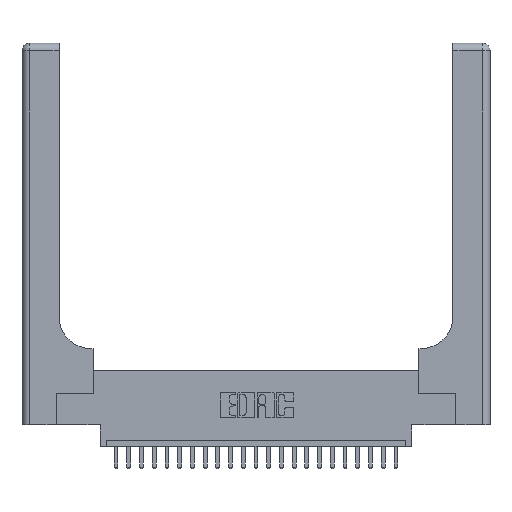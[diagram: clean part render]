
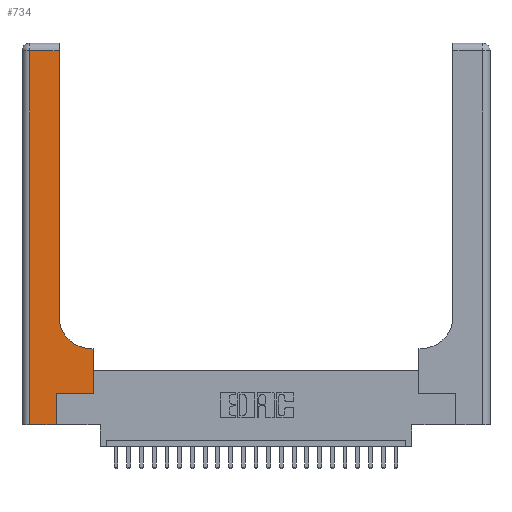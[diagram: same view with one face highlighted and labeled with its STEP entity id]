
A CAD part, top view. The second image highlights one B-rep face of the part: STEP entity #734.
In plain terms, the highlighted planar face has unit normal (0, 0, 1).
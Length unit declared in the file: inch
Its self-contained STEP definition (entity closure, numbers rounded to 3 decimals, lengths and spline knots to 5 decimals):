
#443 = ORIENTED_EDGE ( 'NONE', *, *, #13530, .T. ) ;
#529 = VECTOR ( 'NONE', #8197, 39.37008 ) ;
#697 = ORIENTED_EDGE ( 'NONE', *, *, #7268, .T. ) ;
#734 = ADVANCED_FACE ( 'NONE', ( #11879 ), #20268, .F. ) ;
#1260 = VERTEX_POINT ( 'NONE', #9228 ) ;
#1275 = DIRECTION ( 'NONE',  ( -1., 0., 0. ) ) ;
#1363 = ORIENTED_EDGE ( 'NONE', *, *, #17161, .T. ) ;
#1904 = EDGE_CURVE ( 'NONE', #24239, #1260, #17369, .T. ) ;
#2392 = CARTESIAN_POINT ( 'NONE',  ( 0.5415, 0.6, 0.37 ) ) ;
#2810 = CARTESIAN_POINT ( 'NONE',  ( 0.06, 3., 0.37 ) ) ;
#2931 = LINE ( 'NONE', #3161, #11792 ) ;
#3161 = CARTESIAN_POINT ( 'NONE',  ( 0., 0., 0.37 ) ) ;
#3208 = CARTESIAN_POINT ( 'NONE',  ( 0.5585, 0.6, 0.37 ) ) ;
#3316 = DIRECTION ( 'NONE',  ( 0., 0., -1. ) ) ;
#3609 = VECTOR ( 'NONE', #6597, 39.37008 ) ;
#4708 = ORIENTED_EDGE ( 'NONE', *, *, #6054, .T. ) ;
#4972 = ORIENTED_EDGE ( 'NONE', *, *, #24014, .T. ) ;
#5376 = CARTESIAN_POINT ( 'NONE',  ( 0.269, 0., 0.37 ) ) ;
#5452 = LINE ( 'NONE', #2810, #3609 ) ;
#5463 = CARTESIAN_POINT ( 'NONE',  ( 0.5585, 0.25, 0.37 ) ) ;
#6054 = EDGE_CURVE ( 'NONE', #8722, #24239, #10647, .T. ) ;
#6098 = LINE ( 'NONE', #8687, #15873 ) ;
#6276 = VECTOR ( 'NONE', #16962, 39.37008 ) ;
#6362 = VERTEX_POINT ( 'NONE', #12364 ) ;
#6374 = DIRECTION ( 'NONE',  ( 0., 0., -1. ) ) ;
#6597 = DIRECTION ( 'NONE',  ( 0., -1., 0. ) ) ;
#6871 = CARTESIAN_POINT ( 'NONE',  ( 0.269, 0., 0.37 ) ) ;
#6943 = CARTESIAN_POINT ( 'NONE',  ( 0.269, 0.25, 0.37 ) ) ;
#6971 = EDGE_CURVE ( 'NONE', #22836, #15444, #21625, .T. ) ;
#7268 = EDGE_CURVE ( 'NONE', #15444, #16836, #19467, .T. ) ;
#7806 = ORIENTED_EDGE ( 'NONE', *, *, #6971, .T. ) ;
#8197 = DIRECTION ( 'NONE',  ( -1., 0., 0. ) ) ;
#8687 = CARTESIAN_POINT ( 'NONE',  ( 0., 2.94, 0.37 ) ) ;
#8722 = VERTEX_POINT ( 'NONE', #3208 ) ;
#8725 = DIRECTION ( 'NONE',  ( 1., 0., 0. ) ) ;
#9228 = CARTESIAN_POINT ( 'NONE',  ( 0.2915, 0.85, 0.37 ) ) ;
#9913 = VERTEX_POINT ( 'NONE', #21121 ) ;
#10647 = LINE ( 'NONE', #19911, #529 ) ;
#10932 = CARTESIAN_POINT ( 'NONE',  ( 0., 3., 0.37 ) ) ;
#11119 = CARTESIAN_POINT ( 'NONE',  ( 0.2915, 3., 0.37 ) ) ;
#11792 = VECTOR ( 'NONE', #20704, 39.37008 ) ;
#11879 = FACE_OUTER_BOUND ( 'NONE', #21944, .T. ) ;
#11937 = ORIENTED_EDGE ( 'NONE', *, *, #1904, .T. ) ;
#12273 = DIRECTION ( 'NONE',  ( 0., 1., 0. ) ) ;
#12331 = CARTESIAN_POINT ( 'NONE',  ( 0.5415, 0.85, 0.37 ) ) ;
#12364 = CARTESIAN_POINT ( 'NONE',  ( 0.06, 0., 0.37 ) ) ;
#13530 = EDGE_CURVE ( 'NONE', #9913, #6362, #5452, .T. ) ;
#13837 = VECTOR ( 'NONE', #12273, 39.37008 ) ;
#15166 = LINE ( 'NONE', #11119, #6276 ) ;
#15444 = VERTEX_POINT ( 'NONE', #22569 ) ;
#15873 = VECTOR ( 'NONE', #22297, 39.37008 ) ;
#16594 = ORIENTED_EDGE ( 'NONE', *, *, #21453, .T. ) ;
#16836 = VERTEX_POINT ( 'NONE', #5463 ) ;
#16962 = DIRECTION ( 'NONE',  ( 0., 1., 0. ) ) ;
#17161 = EDGE_CURVE ( 'NONE', #16836, #8722, #17829, .T. ) ;
#17369 = CIRCLE ( 'NONE', #18002, 0.25 ) ;
#17829 = LINE ( 'NONE', #20081, #13837 ) ;
#18002 = AXIS2_PLACEMENT_3D ( 'NONE', #12331, #6374, #22186 ) ;
#19467 = LINE ( 'NONE', #6943, #22539 ) ;
#19479 = CARTESIAN_POINT ( 'NONE',  ( 0.2915, 2.94, 0.37 ) ) ;
#19911 = CARTESIAN_POINT ( 'NONE',  ( 0.2915, 0.6, 0.37 ) ) ;
#20023 = EDGE_CURVE ( 'NONE', #22973, #9913, #6098, .T. ) ;
#20081 = CARTESIAN_POINT ( 'NONE',  ( 0.5585, 0.25, 0.37 ) ) ;
#20268 = PLANE ( 'NONE',  #24662 ) ;
#20704 = DIRECTION ( 'NONE',  ( 1., 0., 0. ) ) ;
#21121 = CARTESIAN_POINT ( 'NONE',  ( 0.06, 2.94, 0.37 ) ) ;
#21177 = ORIENTED_EDGE ( 'NONE', *, *, #20023, .T. ) ;
#21453 = EDGE_CURVE ( 'NONE', #6362, #22836, #2931, .T. ) ;
#21625 = LINE ( 'NONE', #6871, #23461 ) ;
#21944 = EDGE_LOOP ( 'NONE', ( #4972, #21177, #443, #16594, #7806, #697, #1363, #4708, #11937 ) ) ;
#22186 = DIRECTION ( 'NONE',  ( 1., 0., 0. ) ) ;
#22297 = DIRECTION ( 'NONE',  ( -1., 0., 0. ) ) ;
#22539 = VECTOR ( 'NONE', #8725, 39.37008 ) ;
#22569 = CARTESIAN_POINT ( 'NONE',  ( 0.269, 0.25, 0.37 ) ) ;
#22679 = DIRECTION ( 'NONE',  ( 0., 1., 0. ) ) ;
#22836 = VERTEX_POINT ( 'NONE', #5376 ) ;
#22973 = VERTEX_POINT ( 'NONE', #19479 ) ;
#23461 = VECTOR ( 'NONE', #22679, 39.37008 ) ;
#24014 = EDGE_CURVE ( 'NONE', #1260, #22973, #15166, .T. ) ;
#24239 = VERTEX_POINT ( 'NONE', #2392 ) ;
#24662 = AXIS2_PLACEMENT_3D ( 'NONE', #10932, #3316, #1275 ) ;
